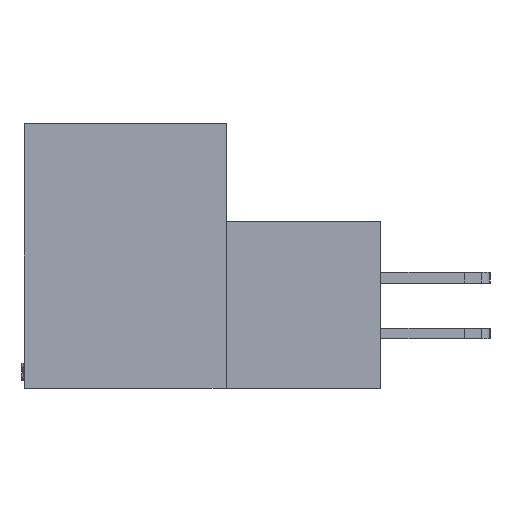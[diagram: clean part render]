
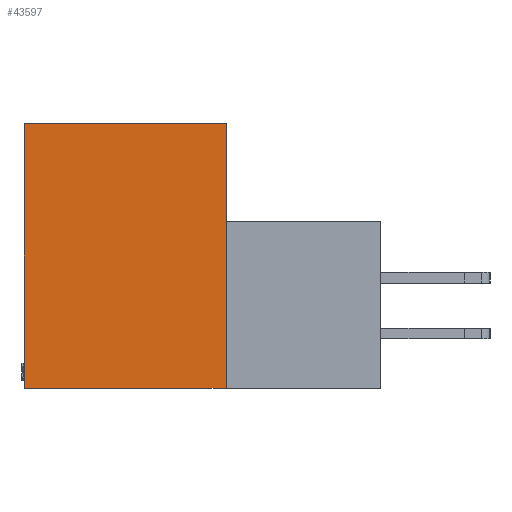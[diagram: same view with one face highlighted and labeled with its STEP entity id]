
A CAD part, left-side view. The second image highlights one B-rep face of the part: STEP entity #43597.
In plain terms, the highlighted planar face has unit normal (-1, 0, 0).
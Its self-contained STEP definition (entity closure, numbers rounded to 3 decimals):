
#373 = CARTESIAN_POINT ( 'NONE',  ( 0., 11.506, 0. ) ) ;
#642 = LINE ( 'NONE', #31429, #6853 ) ;
#1151 = DIRECTION ( 'NONE',  ( 0., 0., -1. ) ) ;
#1774 = VERTEX_POINT ( 'NONE', #11512 ) ;
#2896 = ORIENTED_EDGE ( 'NONE', *, *, #49741, .F. ) ;
#4400 = DIRECTION ( 'NONE',  ( 0., 0., 1. ) ) ;
#5796 = LINE ( 'NONE', #43703, #25581 ) ;
#6853 = VECTOR ( 'NONE', #1151, 1000. ) ;
#7258 = LINE ( 'NONE', #373, #7871 ) ;
#7871 = VECTOR ( 'NONE', #35968, 1000. ) ;
#11512 = CARTESIAN_POINT ( 'NONE',  ( 0., 0., -15.088 ) ) ;
#12233 = CARTESIAN_POINT ( 'NONE',  ( 0., 11.506, 0. ) ) ;
#12449 = VERTEX_POINT ( 'NONE', #48323 ) ;
#14968 = VERTEX_POINT ( 'NONE', #44946 ) ;
#16714 = EDGE_CURVE ( 'NONE', #14968, #21432, #5796, .T. ) ;
#18001 = DIRECTION ( 'NONE',  ( 0., 1., 0. ) ) ;
#18900 = EDGE_CURVE ( 'NONE', #12449, #1774, #642, .T. ) ;
#21432 = VERTEX_POINT ( 'NONE', #12233 ) ;
#22090 = AXIS2_PLACEMENT_3D ( 'NONE', #24190, #48148, #36302 ) ;
#24190 = CARTESIAN_POINT ( 'NONE',  ( 0., 0., 0. ) ) ;
#25581 = VECTOR ( 'NONE', #4400, 1000. ) ;
#29006 = VECTOR ( 'NONE', #18001, 1000. ) ;
#29721 = ORIENTED_EDGE ( 'NONE', *, *, #16714, .F. ) ;
#30234 = CARTESIAN_POINT ( 'NONE',  ( 0., -8.814, -15.088 ) ) ;
#31429 = CARTESIAN_POINT ( 'NONE',  ( 0., 0., 0. ) ) ;
#35838 = LINE ( 'NONE', #30234, #29006 ) ;
#35968 = DIRECTION ( 'NONE',  ( 0., -1., 0. ) ) ;
#36302 = DIRECTION ( 'NONE',  ( 0., 0., -1. ) ) ;
#41137 = EDGE_LOOP ( 'NONE', ( #50163, #42474, #2896, #29721 ) ) ;
#42474 = ORIENTED_EDGE ( 'NONE', *, *, #18900, .F. ) ;
#43597 = ADVANCED_FACE ( 'NONE', ( #49807 ), #44142, .F. ) ;
#43703 = CARTESIAN_POINT ( 'NONE',  ( 0., 11.506, -15.088 ) ) ;
#44142 = PLANE ( 'NONE',  #22090 ) ;
#44946 = CARTESIAN_POINT ( 'NONE',  ( 0., 11.506, -15.088 ) ) ;
#47120 = EDGE_CURVE ( 'NONE', #1774, #14968, #35838, .T. ) ;
#48148 = DIRECTION ( 'NONE',  ( 1., 0., 0. ) ) ;
#48323 = CARTESIAN_POINT ( 'NONE',  ( 0., 0., 0. ) ) ;
#49741 = EDGE_CURVE ( 'NONE', #21432, #12449, #7258, .T. ) ;
#49807 = FACE_OUTER_BOUND ( 'NONE', #41137, .T. ) ;
#50163 = ORIENTED_EDGE ( 'NONE', *, *, #47120, .F. ) ;
